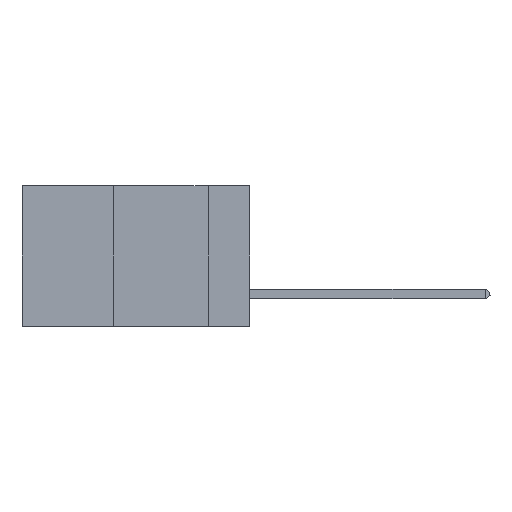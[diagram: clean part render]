
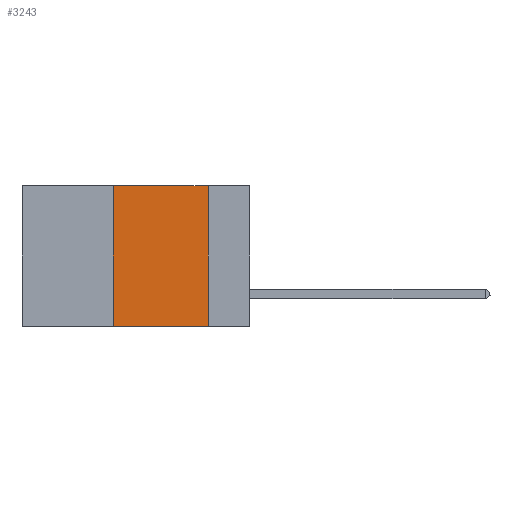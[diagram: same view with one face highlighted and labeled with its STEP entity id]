
A CAD part, left-side view. The second image highlights one B-rep face of the part: STEP entity #3243.
In plain terms, the highlighted planar face has unit normal (-1, 0, 0).
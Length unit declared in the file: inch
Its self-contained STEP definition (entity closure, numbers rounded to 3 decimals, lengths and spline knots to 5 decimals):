
#86 = VERTEX_POINT ( 'NONE', #10836 ) ;
#1141 = EDGE_CURVE ( 'NONE', #86, #15854, #11568, .T. ) ;
#1505 = EDGE_LOOP ( 'NONE', ( #14784, #10996, #8195, #7164 ) ) ;
#2239 = CARTESIAN_POINT ( 'NONE',  ( 0., 0.36, 0. ) ) ;
#2782 = CARTESIAN_POINT ( 'NONE',  ( 0., 0.6, 0. ) ) ;
#3172 = LINE ( 'NONE', #5747, #3644 ) ;
#3181 = VECTOR ( 'NONE', #17816, 39.37008 ) ;
#3243 = ADVANCED_FACE ( 'NONE', ( #6193 ), #17186, .F. ) ;
#3644 = VECTOR ( 'NONE', #10386, 39.37008 ) ;
#5499 = EDGE_CURVE ( 'NONE', #15854, #7003, #3172, .T. ) ;
#5747 = CARTESIAN_POINT ( 'NONE',  ( 0., 0.11, 0. ) ) ;
#6193 = FACE_OUTER_BOUND ( 'NONE', #1505, .T. ) ;
#7003 = VERTEX_POINT ( 'NONE', #18018 ) ;
#7164 = ORIENTED_EDGE ( 'NONE', *, *, #18451, .T. ) ;
#7267 = DIRECTION ( 'NONE',  ( 0., -1., 0. ) ) ;
#7702 = VECTOR ( 'NONE', #12344, 39.37008 ) ;
#8195 = ORIENTED_EDGE ( 'NONE', *, *, #11115, .F. ) ;
#8485 = LINE ( 'NONE', #10456, #9674 ) ;
#9018 = LINE ( 'NONE', #2239, #3181 ) ;
#9674 = VECTOR ( 'NONE', #7267, 39.37008 ) ;
#10386 = DIRECTION ( 'NONE',  ( 0., 0., -1. ) ) ;
#10456 = CARTESIAN_POINT ( 'NONE',  ( 0., 0.6, -0.37 ) ) ;
#10836 = CARTESIAN_POINT ( 'NONE',  ( 0., 0.36, 0. ) ) ;
#10943 = DIRECTION ( 'NONE',  ( 0., 0., -1. ) ) ;
#10996 = ORIENTED_EDGE ( 'NONE', *, *, #1141, .F. ) ;
#11115 = EDGE_CURVE ( 'NONE', #17092, #86, #9018, .T. ) ;
#11568 = LINE ( 'NONE', #2782, #7702 ) ;
#12344 = DIRECTION ( 'NONE',  ( 0., -1., 0. ) ) ;
#12835 = AXIS2_PLACEMENT_3D ( 'NONE', #15574, #17247, #10943 ) ;
#14784 = ORIENTED_EDGE ( 'NONE', *, *, #5499, .F. ) ;
#15574 = CARTESIAN_POINT ( 'NONE',  ( 0., 0.6, 0. ) ) ;
#15854 = VERTEX_POINT ( 'NONE', #18253 ) ;
#17092 = VERTEX_POINT ( 'NONE', #17863 ) ;
#17186 = PLANE ( 'NONE',  #12835 ) ;
#17247 = DIRECTION ( 'NONE',  ( 1., 0., 0. ) ) ;
#17816 = DIRECTION ( 'NONE',  ( 0., 0., 1. ) ) ;
#17863 = CARTESIAN_POINT ( 'NONE',  ( 0., 0.36, -0.37 ) ) ;
#18018 = CARTESIAN_POINT ( 'NONE',  ( 0., 0.11, -0.37 ) ) ;
#18253 = CARTESIAN_POINT ( 'NONE',  ( 0., 0.11, 0. ) ) ;
#18451 = EDGE_CURVE ( 'NONE', #17092, #7003, #8485, .T. ) ;
